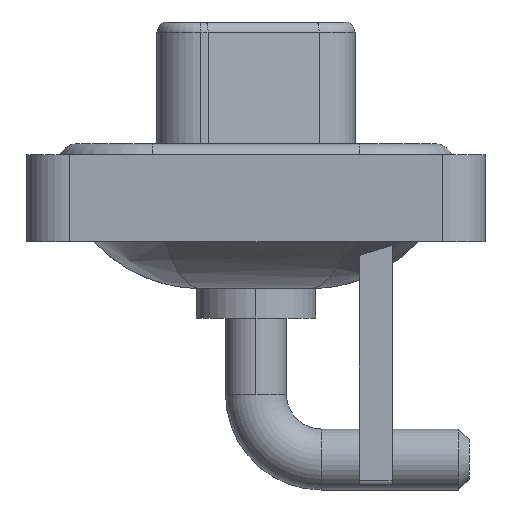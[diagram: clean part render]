
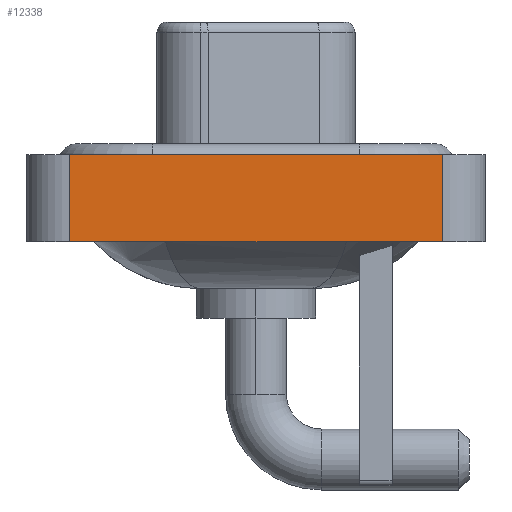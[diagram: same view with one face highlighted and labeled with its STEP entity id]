
A CAD part, left-side view. The second image highlights one B-rep face of the part: STEP entity #12338.
In plain terms, the highlighted planar face has unit normal (-1, 0, 0).
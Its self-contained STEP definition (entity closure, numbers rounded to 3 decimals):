
#184 = LINE ( 'NONE', #1819, #752 ) ;
#717 = VECTOR ( 'NONE', #13976, 1000. ) ;
#752 = VECTOR ( 'NONE', #14843, 1000. ) ;
#1003 = CARTESIAN_POINT ( 'NONE',  ( -7.3, -8.55, 0.4 ) ) ;
#1242 = CARTESIAN_POINT ( 'NONE',  ( -7.3, 8.55, 0.4 ) ) ;
#1665 = EDGE_CURVE ( 'NONE', #11477, #14914, #11782, .T. ) ;
#1819 = CARTESIAN_POINT ( 'NONE',  ( -7.3, -8.55, 0.4 ) ) ;
#2032 = EDGE_CURVE ( 'NONE', #11340, #11477, #3389, .T. ) ;
#2230 = ORIENTED_EDGE ( 'NONE', *, *, #1665, .T. ) ;
#2422 = AXIS2_PLACEMENT_3D ( 'NONE', #9205, #14693, #5459 ) ;
#3077 = VERTEX_POINT ( 'NONE', #1242 ) ;
#3389 = LINE ( 'NONE', #13698, #12737 ) ;
#4533 = DIRECTION ( 'NONE',  ( 0., -1., 0. ) ) ;
#4666 = LINE ( 'NONE', #10235, #717 ) ;
#4742 = CARTESIAN_POINT ( 'NONE',  ( -7.3, -8.55, -3.6 ) ) ;
#5167 = CARTESIAN_POINT ( 'NONE',  ( -7.3, -8.55, -3.6 ) ) ;
#5459 = DIRECTION ( 'NONE',  ( 0., 0., 1. ) ) ;
#6857 = PLANE ( 'NONE',  #2422 ) ;
#6909 = VECTOR ( 'NONE', #13285, 1000. ) ;
#6961 = EDGE_CURVE ( 'NONE', #11340, #3077, #4666, .T. ) ;
#7219 = EDGE_LOOP ( 'NONE', ( #2230, #16894, #8322, #8034 ) ) ;
#7982 = FACE_OUTER_BOUND ( 'NONE', #7219, .T. ) ;
#8034 = ORIENTED_EDGE ( 'NONE', *, *, #2032, .T. ) ;
#8322 = ORIENTED_EDGE ( 'NONE', *, *, #6961, .F. ) ;
#9205 = CARTESIAN_POINT ( 'NONE',  ( -7.3, -8.55, -3.6 ) ) ;
#10235 = CARTESIAN_POINT ( 'NONE',  ( -7.3, 8.55, -3.6 ) ) ;
#11340 = VERTEX_POINT ( 'NONE', #13897 ) ;
#11477 = VERTEX_POINT ( 'NONE', #4742 ) ;
#11782 = LINE ( 'NONE', #5167, #6909 ) ;
#12338 = ADVANCED_FACE ( 'NONE', ( #7982 ), #6857, .T. ) ;
#12737 = VECTOR ( 'NONE', #4533, 1000. ) ;
#12827 = EDGE_CURVE ( 'NONE', #3077, #14914, #184, .T. ) ;
#13285 = DIRECTION ( 'NONE',  ( 0., 0., 1. ) ) ;
#13698 = CARTESIAN_POINT ( 'NONE',  ( -7.3, -8.55, -3.6 ) ) ;
#13897 = CARTESIAN_POINT ( 'NONE',  ( -7.3, 8.55, -3.6 ) ) ;
#13976 = DIRECTION ( 'NONE',  ( 0., 0., 1. ) ) ;
#14693 = DIRECTION ( 'NONE',  ( -1., 0., 0. ) ) ;
#14843 = DIRECTION ( 'NONE',  ( 0., -1., 0. ) ) ;
#14914 = VERTEX_POINT ( 'NONE', #1003 ) ;
#16894 = ORIENTED_EDGE ( 'NONE', *, *, #12827, .F. ) ;
